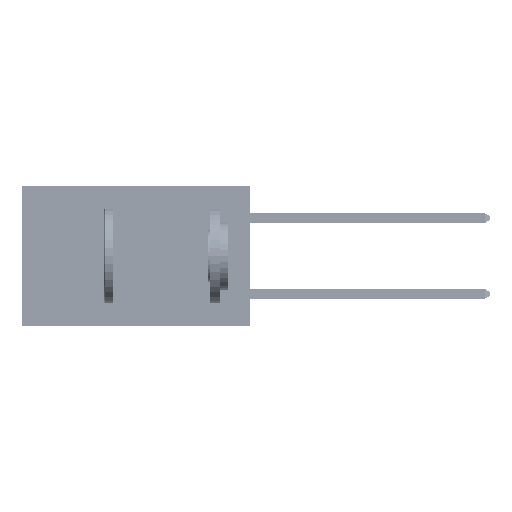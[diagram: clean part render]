
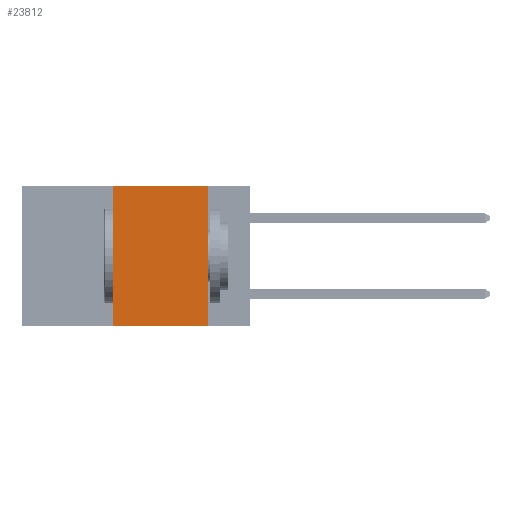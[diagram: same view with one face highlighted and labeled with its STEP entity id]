
A CAD part, left-side view. The second image highlights one B-rep face of the part: STEP entity #23812.
In plain terms, the highlighted planar face has unit normal (-1, 0, 0).
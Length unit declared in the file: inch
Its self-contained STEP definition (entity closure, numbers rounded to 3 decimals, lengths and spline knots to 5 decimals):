
#1415 = LINE ( 'NONE', #5151, #18612 ) ;
#1916 = PLANE ( 'NONE',  #16566 ) ;
#3733 = DIRECTION ( 'NONE',  ( 0., 0., 1. ) ) ;
#3999 = DIRECTION ( 'NONE',  ( 0., 0., -1. ) ) ;
#4015 = ORIENTED_EDGE ( 'NONE', *, *, #10535, .T. ) ;
#4574 = VERTEX_POINT ( 'NONE', #13161 ) ;
#5151 = CARTESIAN_POINT ( 'NONE',  ( 0., 0.6, -0.37 ) ) ;
#6194 = CARTESIAN_POINT ( 'NONE',  ( 0., 0.6, 0. ) ) ;
#10535 = EDGE_CURVE ( 'NONE', #12398, #24200, #1415, .T. ) ;
#10842 = ORIENTED_EDGE ( 'NONE', *, *, #41208, .F. ) ;
#11461 = CARTESIAN_POINT ( 'NONE',  ( 0., 0.36, 0. ) ) ;
#12047 = ORIENTED_EDGE ( 'NONE', *, *, #48437, .F. ) ;
#12398 = VERTEX_POINT ( 'NONE', #17288 ) ;
#13161 = CARTESIAN_POINT ( 'NONE',  ( 0., 0.11, 0. ) ) ;
#13561 = ORIENTED_EDGE ( 'NONE', *, *, #16114, .F. ) ;
#15676 = VECTOR ( 'NONE', #3999, 39.37008 ) ;
#15989 = CARTESIAN_POINT ( 'NONE',  ( 0., 0.36, 0. ) ) ;
#16114 = EDGE_CURVE ( 'NONE', #4574, #24200, #18829, .T. ) ;
#16566 = AXIS2_PLACEMENT_3D ( 'NONE', #6194, #30868, #42680 ) ;
#17288 = CARTESIAN_POINT ( 'NONE',  ( 0., 0.36, -0.37 ) ) ;
#18612 = VECTOR ( 'NONE', #36984, 39.37008 ) ;
#18829 = LINE ( 'NONE', #48651, #15676 ) ;
#21237 = VERTEX_POINT ( 'NONE', #11461 ) ;
#23812 = ADVANCED_FACE ( 'NONE', ( #47894 ), #1916, .F. ) ;
#24200 = VERTEX_POINT ( 'NONE', #49531 ) ;
#28793 = EDGE_LOOP ( 'NONE', ( #13561, #10842, #12047, #4015 ) ) ;
#30868 = DIRECTION ( 'NONE',  ( 1., 0., 0. ) ) ;
#36241 = DIRECTION ( 'NONE',  ( 0., -1., 0. ) ) ;
#36594 = CARTESIAN_POINT ( 'NONE',  ( 0., 0.6, 0. ) ) ;
#36984 = DIRECTION ( 'NONE',  ( 0., -1., 0. ) ) ;
#41208 = EDGE_CURVE ( 'NONE', #21237, #4574, #48473, .T. ) ;
#42680 = DIRECTION ( 'NONE',  ( 0., 0., -1. ) ) ;
#43781 = LINE ( 'NONE', #15989, #48219 ) ;
#47866 = VECTOR ( 'NONE', #36241, 39.37008 ) ;
#47894 = FACE_OUTER_BOUND ( 'NONE', #28793, .T. ) ;
#48219 = VECTOR ( 'NONE', #3733, 39.37008 ) ;
#48437 = EDGE_CURVE ( 'NONE', #12398, #21237, #43781, .T. ) ;
#48473 = LINE ( 'NONE', #36594, #47866 ) ;
#48651 = CARTESIAN_POINT ( 'NONE',  ( 0., 0.11, 0. ) ) ;
#49531 = CARTESIAN_POINT ( 'NONE',  ( 0., 0.11, -0.37 ) ) ;
